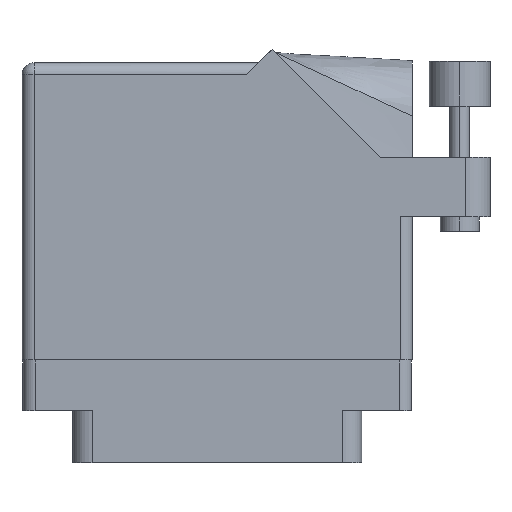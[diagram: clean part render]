
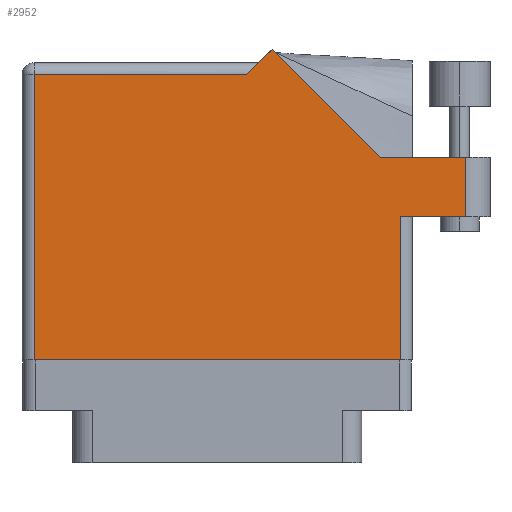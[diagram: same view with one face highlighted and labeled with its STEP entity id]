
A CAD part, front view. The second image highlights one B-rep face of the part: STEP entity #2952.
In plain terms, the highlighted face is planar.
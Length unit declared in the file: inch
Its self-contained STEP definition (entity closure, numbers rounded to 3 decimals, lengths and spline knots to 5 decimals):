
#790 = DIRECTION ( 'NONE',  ( 0., -1., 0. ) ) ;
#1350 = LINE ( 'NONE', #20519, #16419 ) ;
#2930 = LINE ( 'NONE', #19322, #37787 ) ;
#2952 = ADVANCED_FACE ( 'NONE', ( #12037 ), #13340, .F. ) ;
#3250 = VERTEX_POINT ( 'NONE', #8710 ) ;
#3274 = ORIENTED_EDGE ( 'NONE', *, *, #3841, .T. ) ;
#3344 = VERTEX_POINT ( 'NONE', #36331 ) ;
#3714 = CARTESIAN_POINT ( 'NONE',  ( 1.84442, 1.044, 0. ) ) ;
#3841 = EDGE_CURVE ( 'NONE', #3344, #12899, #21344, .T. ) ;
#4234 = CARTESIAN_POINT ( 'NONE',  ( 0.062, 0., 0. ) ) ;
#4496 = ORIENTED_EDGE ( 'NONE', *, *, #11261, .T. ) ;
#4764 = DIRECTION ( 'NONE',  ( -1., 0., 0. ) ) ;
#5639 = EDGE_CURVE ( 'NONE', #3250, #29557, #2930, .T. ) ;
#5695 = VECTOR ( 'NONE', #6171, 39.37008 ) ;
#5751 = CARTESIAN_POINT ( 'NONE',  ( 2.285, 0.737, 0. ) ) ;
#5874 = ORIENTED_EDGE ( 'NONE', *, *, #12184, .T. ) ;
#6040 = CARTESIAN_POINT ( 'NONE',  ( 2.01, 0.737, 0. ) ) ;
#6171 = DIRECTION ( 'NONE',  ( 1., 0., 0. ) ) ;
#6271 = CARTESIAN_POINT ( 'NONE',  ( 1.948, 0.737, 0. ) ) ;
#7557 = LINE ( 'NONE', #19582, #38625 ) ;
#7844 = ORIENTED_EDGE ( 'NONE', *, *, #35461, .T. ) ;
#8710 = CARTESIAN_POINT ( 'NONE',  ( 0.062, 1.468, 0. ) ) ;
#10167 = DIRECTION ( 'NONE',  ( -0.707, 0.707, 0. ) ) ;
#11261 = EDGE_CURVE ( 'NONE', #29557, #3344, #26344, .T. ) ;
#12037 = FACE_OUTER_BOUND ( 'NONE', #32861, .T. ) ;
#12184 = EDGE_CURVE ( 'NONE', #25366, #15377, #1350, .T. ) ;
#12899 = VERTEX_POINT ( 'NONE', #6271 ) ;
#13207 = VECTOR ( 'NONE', #34982, 39.37008 ) ;
#13214 = DIRECTION ( 'NONE',  ( 0., 1., 0. ) ) ;
#13340 = PLANE ( 'NONE',  #21443 ) ;
#13829 = ORIENTED_EDGE ( 'NONE', *, *, #21174, .T. ) ;
#14269 = VERTEX_POINT ( 'NONE', #29517 ) ;
#14407 = LINE ( 'NONE', #19327, #28525 ) ;
#15377 = VERTEX_POINT ( 'NONE', #31174 ) ;
#15836 = ORIENTED_EDGE ( 'NONE', *, *, #34469, .T. ) ;
#16419 = VECTOR ( 'NONE', #23662, 39.37008 ) ;
#16433 = VERTEX_POINT ( 'NONE', #17487 ) ;
#17487 = CARTESIAN_POINT ( 'NONE',  ( 1.84442, 1.044, 0. ) ) ;
#18926 = DIRECTION ( 'NONE',  ( -1., 0., 0. ) ) ;
#19246 = DIRECTION ( 'NONE',  ( 0., 0., -1. ) ) ;
#19322 = CARTESIAN_POINT ( 'NONE',  ( 0.062, 0., 0. ) ) ;
#19327 = CARTESIAN_POINT ( 'NONE',  ( 2.41, 1.044, 0. ) ) ;
#19582 = CARTESIAN_POINT ( 'NONE',  ( 0., 1.468, 0. ) ) ;
#20291 = DIRECTION ( 'NONE',  ( 0., 1., 0. ) ) ;
#20519 = CARTESIAN_POINT ( 'NONE',  ( 1.217, 1.53, 0. ) ) ;
#20651 = VECTOR ( 'NONE', #10167, 39.37008 ) ;
#20894 = LINE ( 'NONE', #31643, #22305 ) ;
#21174 = EDGE_CURVE ( 'NONE', #14269, #16433, #14407, .T. ) ;
#21344 = LINE ( 'NONE', #38329, #25120 ) ;
#21443 = AXIS2_PLACEMENT_3D ( 'NONE', #28196, #19246, #4764 ) ;
#22305 = VECTOR ( 'NONE', #13214, 39.37008 ) ;
#22466 = EDGE_CURVE ( 'NONE', #31844, #14269, #20894, .T. ) ;
#22732 = CARTESIAN_POINT ( 'NONE',  ( 0., 0., 0. ) ) ;
#23662 = DIRECTION ( 'NONE',  ( -0.707, -0.707, 0. ) ) ;
#24517 = LINE ( 'NONE', #6040, #5695 ) ;
#25120 = VECTOR ( 'NONE', #20291, 39.37008 ) ;
#25366 = VERTEX_POINT ( 'NONE', #33318 ) ;
#25466 = ORIENTED_EDGE ( 'NONE', *, *, #27892, .T. ) ;
#26025 = ORIENTED_EDGE ( 'NONE', *, *, #5639, .T. ) ;
#26344 = LINE ( 'NONE', #22732, #13207 ) ;
#27892 = EDGE_CURVE ( 'NONE', #12899, #31844, #24517, .T. ) ;
#27942 = ORIENTED_EDGE ( 'NONE', *, *, #22466, .T. ) ;
#28196 = CARTESIAN_POINT ( 'NONE',  ( 0., 1.53, 0. ) ) ;
#28378 = DIRECTION ( 'NONE',  ( -1., 0., 0. ) ) ;
#28525 = VECTOR ( 'NONE', #18926, 39.37008 ) ;
#29517 = CARTESIAN_POINT ( 'NONE',  ( 2.285, 1.044, 0. ) ) ;
#29557 = VERTEX_POINT ( 'NONE', #4234 ) ;
#31174 = CARTESIAN_POINT ( 'NONE',  ( 1.155, 1.468, 0. ) ) ;
#31643 = CARTESIAN_POINT ( 'NONE',  ( 2.285, 1.044, 0. ) ) ;
#31844 = VERTEX_POINT ( 'NONE', #5751 ) ;
#32861 = EDGE_LOOP ( 'NONE', ( #25466, #27942, #13829, #7844, #5874, #15836, #26025, #4496, #3274 ) ) ;
#33318 = CARTESIAN_POINT ( 'NONE',  ( 1.28771, 1.60071, 0. ) ) ;
#34469 = EDGE_CURVE ( 'NONE', #15377, #3250, #7557, .T. ) ;
#34982 = DIRECTION ( 'NONE',  ( 1., 0., 0. ) ) ;
#35461 = EDGE_CURVE ( 'NONE', #16433, #25366, #37139, .T. ) ;
#36331 = CARTESIAN_POINT ( 'NONE',  ( 1.948, 0., 0. ) ) ;
#37139 = LINE ( 'NONE', #3714, #20651 ) ;
#37787 = VECTOR ( 'NONE', #790, 39.37008 ) ;
#38329 = CARTESIAN_POINT ( 'NONE',  ( 1.948, 0.737, 0. ) ) ;
#38625 = VECTOR ( 'NONE', #28378, 39.37008 ) ;
